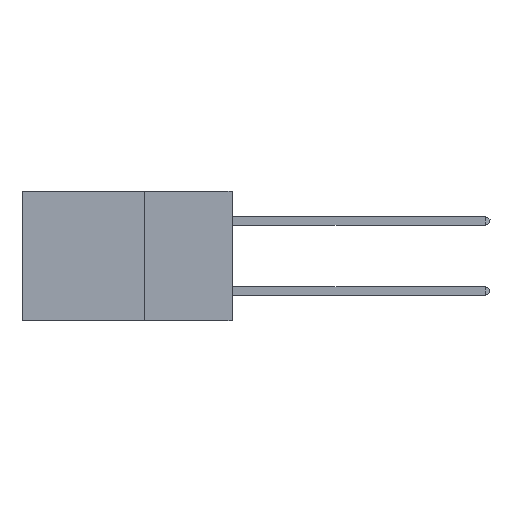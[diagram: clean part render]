
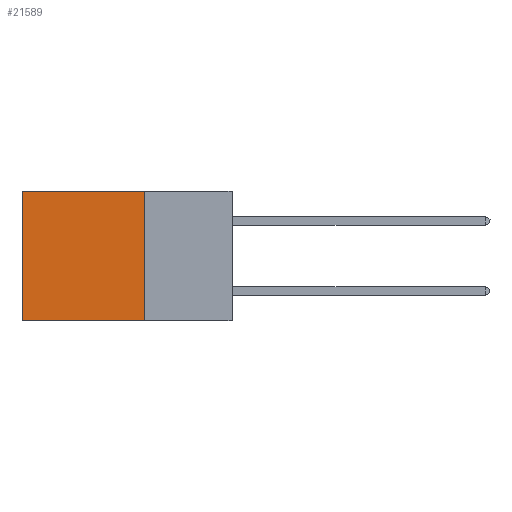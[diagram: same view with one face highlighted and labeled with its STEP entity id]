
A CAD part, left-side view. The second image highlights one B-rep face of the part: STEP entity #21589.
In plain terms, the highlighted planar face has unit normal (-1, 0, 0).
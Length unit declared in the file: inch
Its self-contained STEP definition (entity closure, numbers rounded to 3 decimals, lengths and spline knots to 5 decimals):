
#48 = LINE ( 'NONE', #31034, #35518 ) ;
#861 = CARTESIAN_POINT ( 'NONE',  ( 0.2875, 0.25, 0. ) ) ;
#1414 = CARTESIAN_POINT ( 'NONE',  ( 0.2875, 0.25, -0.37 ) ) ;
#1562 = VERTEX_POINT ( 'NONE', #21692 ) ;
#2072 = EDGE_CURVE ( 'NONE', #1562, #27586, #14507, .T. ) ;
#4217 = DIRECTION ( 'NONE',  ( 1., 0., 0. ) ) ;
#8680 = CARTESIAN_POINT ( 'NONE',  ( 0.2875, 0.6, -0.37 ) ) ;
#9228 = EDGE_LOOP ( 'NONE', ( #41092, #17146, #30169, #14908 ) ) ;
#14291 = DIRECTION ( 'NONE',  ( 0., 0., -1. ) ) ;
#14491 = CARTESIAN_POINT ( 'NONE',  ( 0.2875, 0.6, 0. ) ) ;
#14507 = LINE ( 'NONE', #861, #25253 ) ;
#14908 = ORIENTED_EDGE ( 'NONE', *, *, #2072, .T. ) ;
#16134 = VECTOR ( 'NONE', #40186, 39.37008 ) ;
#17146 = ORIENTED_EDGE ( 'NONE', *, *, #33276, .F. ) ;
#17370 = LINE ( 'NONE', #26546, #35689 ) ;
#18054 = AXIS2_PLACEMENT_3D ( 'NONE', #24337, #4217, #14291 ) ;
#18790 = VERTEX_POINT ( 'NONE', #1414 ) ;
#20694 = DIRECTION ( 'NONE',  ( 0., 0., -1. ) ) ;
#21589 = ADVANCED_FACE ( 'NONE', ( #43227 ), #41925, .F. ) ;
#21692 = CARTESIAN_POINT ( 'NONE',  ( 0.2875, 0.25, 0. ) ) ;
#23249 = DIRECTION ( 'NONE',  ( 0., 1., 0. ) ) ;
#24337 = CARTESIAN_POINT ( 'NONE',  ( 0.2875, 0.25, 0. ) ) ;
#25238 = LINE ( 'NONE', #26618, #16134 ) ;
#25253 = VECTOR ( 'NONE', #42307, 39.37008 ) ;
#26546 = CARTESIAN_POINT ( 'NONE',  ( 0.2875, 0.25, -0.37 ) ) ;
#26618 = CARTESIAN_POINT ( 'NONE',  ( 0.2875, 0.6, 0. ) ) ;
#27586 = VERTEX_POINT ( 'NONE', #14491 ) ;
#30169 = ORIENTED_EDGE ( 'NONE', *, *, #35181, .F. ) ;
#30955 = VERTEX_POINT ( 'NONE', #8680 ) ;
#31034 = CARTESIAN_POINT ( 'NONE',  ( 0.2875, 0.25, 0. ) ) ;
#33276 = EDGE_CURVE ( 'NONE', #18790, #30955, #17370, .T. ) ;
#35181 = EDGE_CURVE ( 'NONE', #1562, #18790, #48, .T. ) ;
#35518 = VECTOR ( 'NONE', #20694, 39.37008 ) ;
#35689 = VECTOR ( 'NONE', #23249, 39.37008 ) ;
#38579 = EDGE_CURVE ( 'NONE', #27586, #30955, #25238, .T. ) ;
#40186 = DIRECTION ( 'NONE',  ( 0., 0., -1. ) ) ;
#41092 = ORIENTED_EDGE ( 'NONE', *, *, #38579, .T. ) ;
#41925 = PLANE ( 'NONE',  #18054 ) ;
#42307 = DIRECTION ( 'NONE',  ( 0., 1., 0. ) ) ;
#43227 = FACE_OUTER_BOUND ( 'NONE', #9228, .T. ) ;
